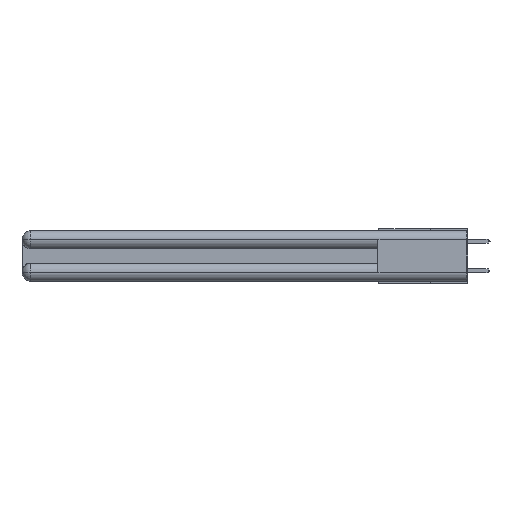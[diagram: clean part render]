
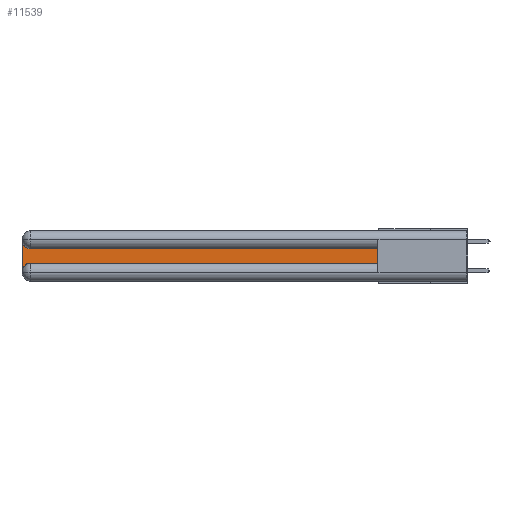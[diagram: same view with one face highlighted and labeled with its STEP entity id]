
A CAD part, left-side view. The second image highlights one B-rep face of the part: STEP entity #11539.
In plain terms, the highlighted planar face has unit normal (-1, 0, 0).
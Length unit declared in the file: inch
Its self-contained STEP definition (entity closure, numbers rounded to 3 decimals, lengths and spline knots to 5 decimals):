
#810 = ORIENTED_EDGE ( 'NONE', *, *, #20014, .T. ) ;
#1302 = DIRECTION ( 'NONE',  ( 0., 0., -1. ) ) ;
#1974 = CIRCLE ( 'NONE', #15059, 0.06 ) ;
#2051 = DIRECTION ( 'NONE',  ( 1., 0., 0. ) ) ;
#2085 = VERTEX_POINT ( 'NONE', #4603 ) ;
#2389 = DIRECTION ( 'NONE',  ( 0., 0., 1. ) ) ;
#2408 = CARTESIAN_POINT ( 'NONE',  ( 0.075, 3., -0.2175 ) ) ;
#2410 = EDGE_CURVE ( 'NONE', #16039, #11956, #22761, .T. ) ;
#4213 = CARTESIAN_POINT ( 'NONE',  ( 0.075, 0.6, -0.2175 ) ) ;
#4603 = CARTESIAN_POINT ( 'NONE',  ( 0.075, 2.94, -0.2175 ) ) ;
#4797 = CARTESIAN_POINT ( 'NONE',  ( 0.075, 0.6, -0.2175 ) ) ;
#4814 = ORIENTED_EDGE ( 'NONE', *, *, #5532, .T. ) ;
#5169 = ORIENTED_EDGE ( 'NONE', *, *, #2410, .T. ) ;
#5196 = CARTESIAN_POINT ( 'NONE',  ( 0.075, 3., -0.2775 ) ) ;
#5435 = DIRECTION ( 'NONE',  ( 0., 0., -1. ) ) ;
#5532 = EDGE_CURVE ( 'NONE', #6012, #2085, #1974, .T. ) ;
#5862 = DIRECTION ( 'NONE',  ( 1., 0., 0. ) ) ;
#6012 = VERTEX_POINT ( 'NONE', #5196 ) ;
#6098 = EDGE_CURVE ( 'NONE', #11956, #9138, #29263, .T. ) ;
#7058 = CARTESIAN_POINT ( 'NONE',  ( 0.075, 2.94, -0.1225 ) ) ;
#9138 = VERTEX_POINT ( 'NONE', #7058 ) ;
#9723 = ORIENTED_EDGE ( 'NONE', *, *, #10738, .T. ) ;
#10738 = EDGE_CURVE ( 'NONE', #12676, #6012, #29030, .T. ) ;
#11258 = DIRECTION ( 'NONE',  ( 0., -1., 0. ) ) ;
#11539 = ADVANCED_FACE ( 'NONE', ( #24224 ), #24986, .F. ) ;
#11956 = VERTEX_POINT ( 'NONE', #24345 ) ;
#12676 = VERTEX_POINT ( 'NONE', #23550 ) ;
#13347 = LINE ( 'NONE', #4213, #29364 ) ;
#13423 = DIRECTION ( 'NONE',  ( 1., 0., 0. ) ) ;
#13549 = DIRECTION ( 'NONE',  ( 0., 1., 0. ) ) ;
#13657 = CARTESIAN_POINT ( 'NONE',  ( 0.075, 0.6, -0.1225 ) ) ;
#14890 = CARTESIAN_POINT ( 'NONE',  ( 0.075, 3., -0.1225 ) ) ;
#15059 = AXIS2_PLACEMENT_3D ( 'NONE', #22479, #5862, #1302 ) ;
#16039 = VERTEX_POINT ( 'NONE', #4797 ) ;
#16087 = DIRECTION ( 'NONE',  ( 0., 0., -1. ) ) ;
#16474 = CIRCLE ( 'NONE', #24006, 0.06 ) ;
#18480 = EDGE_LOOP ( 'NONE', ( #20586, #810, #9723, #4814, #22801, #5169 ) ) ;
#20014 = EDGE_CURVE ( 'NONE', #9138, #12676, #16474, .T. ) ;
#20586 = ORIENTED_EDGE ( 'NONE', *, *, #6098, .T. ) ;
#22060 = VECTOR ( 'NONE', #28033, 39.37008 ) ;
#22293 = VECTOR ( 'NONE', #13549, 39.37008 ) ;
#22479 = CARTESIAN_POINT ( 'NONE',  ( 0.075, 2.94, -0.2775 ) ) ;
#22761 = LINE ( 'NONE', #23701, #25677 ) ;
#22801 = ORIENTED_EDGE ( 'NONE', *, *, #26276, .T. ) ;
#23550 = CARTESIAN_POINT ( 'NONE',  ( 0.075, 3., -0.0625 ) ) ;
#23701 = CARTESIAN_POINT ( 'NONE',  ( 0.075, 0.6, -0.2175 ) ) ;
#24006 = AXIS2_PLACEMENT_3D ( 'NONE', #27481, #2051, #16087 ) ;
#24224 = FACE_OUTER_BOUND ( 'NONE', #18480, .T. ) ;
#24345 = CARTESIAN_POINT ( 'NONE',  ( 0.075, 0.6, -0.1225 ) ) ;
#24448 = AXIS2_PLACEMENT_3D ( 'NONE', #14890, #13423, #5435 ) ;
#24986 = PLANE ( 'NONE',  #24448 ) ;
#25677 = VECTOR ( 'NONE', #2389, 39.37008 ) ;
#26276 = EDGE_CURVE ( 'NONE', #2085, #16039, #13347, .T. ) ;
#27481 = CARTESIAN_POINT ( 'NONE',  ( 0.075, 2.94, -0.0625 ) ) ;
#28033 = DIRECTION ( 'NONE',  ( 0., 0., -1. ) ) ;
#29030 = LINE ( 'NONE', #2408, #22060 ) ;
#29263 = LINE ( 'NONE', #13657, #22293 ) ;
#29364 = VECTOR ( 'NONE', #11258, 39.37008 ) ;
